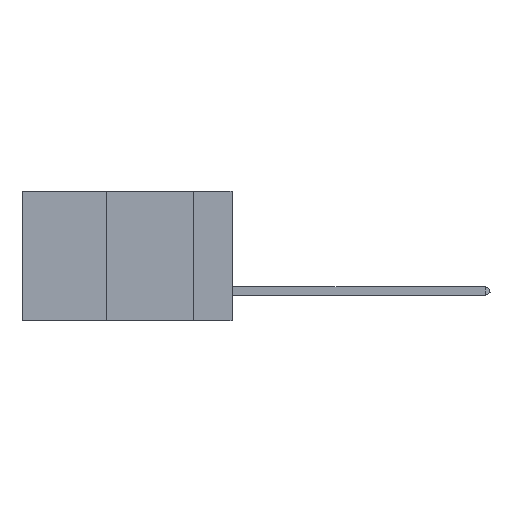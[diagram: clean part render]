
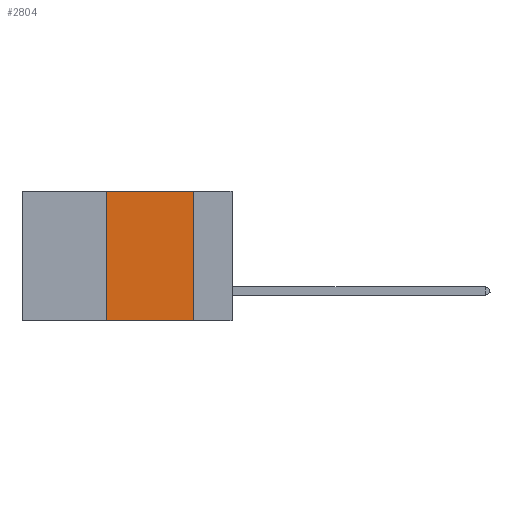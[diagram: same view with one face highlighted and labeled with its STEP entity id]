
A CAD part, left-side view. The second image highlights one B-rep face of the part: STEP entity #2804.
In plain terms, the highlighted planar face has unit normal (-1, 0, 0).
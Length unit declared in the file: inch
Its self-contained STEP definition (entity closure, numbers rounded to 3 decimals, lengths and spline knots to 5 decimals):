
#51 = DIRECTION ( 'NONE',  ( 0., -1., 0. ) ) ;
#193 = DIRECTION ( 'NONE',  ( 0., 0., -1. ) ) ;
#874 = FACE_OUTER_BOUND ( 'NONE', #1247, .T. ) ;
#944 = CARTESIAN_POINT ( 'NONE',  ( 0., 0.6, 0. ) ) ;
#948 = VECTOR ( 'NONE', #193, 39.37008 ) ;
#1247 = EDGE_LOOP ( 'NONE', ( #4116, #1807, #11623, #7985 ) ) ;
#1330 = DIRECTION ( 'NONE',  ( 0., 0., 1. ) ) ;
#1807 = ORIENTED_EDGE ( 'NONE', *, *, #3514, .F. ) ;
#2804 = ADVANCED_FACE ( 'NONE', ( #874 ), #4095, .F. ) ;
#3027 = CARTESIAN_POINT ( 'NONE',  ( 0., 0.6, 0. ) ) ;
#3146 = CARTESIAN_POINT ( 'NONE',  ( 0., 0.6, -0.37 ) ) ;
#3514 = EDGE_CURVE ( 'NONE', #6496, #11030, #12926, .T. ) ;
#3750 = CARTESIAN_POINT ( 'NONE',  ( 0., 0.36, -0.37 ) ) ;
#4095 = PLANE ( 'NONE',  #4338 ) ;
#4116 = ORIENTED_EDGE ( 'NONE', *, *, #7082, .F. ) ;
#4338 = AXIS2_PLACEMENT_3D ( 'NONE', #944, #5091, #6118 ) ;
#5052 = CARTESIAN_POINT ( 'NONE',  ( 0., 0.11, 0. ) ) ;
#5091 = DIRECTION ( 'NONE',  ( 1., 0., 0. ) ) ;
#5309 = CARTESIAN_POINT ( 'NONE',  ( 0., 0.36, 0. ) ) ;
#6118 = DIRECTION ( 'NONE',  ( 0., 0., -1. ) ) ;
#6496 = VERTEX_POINT ( 'NONE', #6594 ) ;
#6594 = CARTESIAN_POINT ( 'NONE',  ( 0., 0.36, 0. ) ) ;
#6727 = VECTOR ( 'NONE', #1330, 39.37008 ) ;
#6838 = VECTOR ( 'NONE', #51, 39.37008 ) ;
#7082 = EDGE_CURVE ( 'NONE', #11030, #12954, #7852, .T. ) ;
#7337 = LINE ( 'NONE', #5309, #6727 ) ;
#7852 = LINE ( 'NONE', #5052, #948 ) ;
#7985 = ORIENTED_EDGE ( 'NONE', *, *, #9145, .T. ) ;
#9045 = DIRECTION ( 'NONE',  ( 0., -1., 0. ) ) ;
#9145 = EDGE_CURVE ( 'NONE', #12034, #12954, #11731, .T. ) ;
#11030 = VERTEX_POINT ( 'NONE', #11953 ) ;
#11405 = CARTESIAN_POINT ( 'NONE',  ( 0., 0.11, -0.37 ) ) ;
#11623 = ORIENTED_EDGE ( 'NONE', *, *, #12424, .F. ) ;
#11731 = LINE ( 'NONE', #3146, #12506 ) ;
#11953 = CARTESIAN_POINT ( 'NONE',  ( 0., 0.11, 0. ) ) ;
#12034 = VERTEX_POINT ( 'NONE', #3750 ) ;
#12424 = EDGE_CURVE ( 'NONE', #12034, #6496, #7337, .T. ) ;
#12506 = VECTOR ( 'NONE', #9045, 39.37008 ) ;
#12926 = LINE ( 'NONE', #3027, #6838 ) ;
#12954 = VERTEX_POINT ( 'NONE', #11405 ) ;
